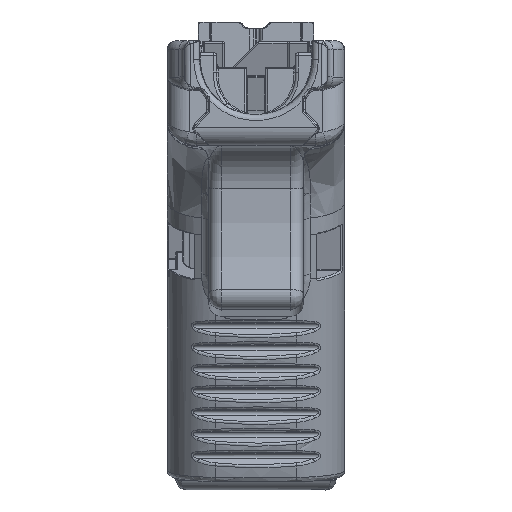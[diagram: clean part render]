
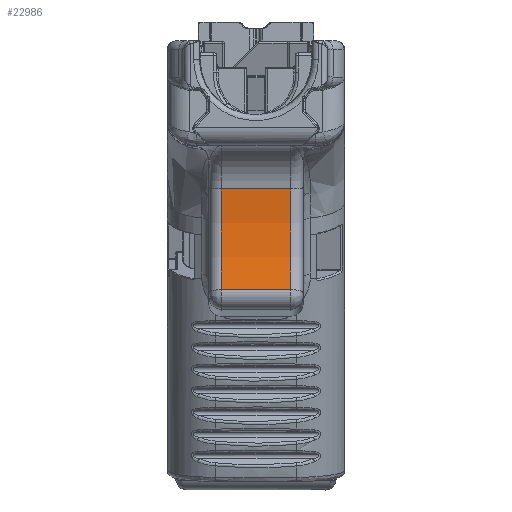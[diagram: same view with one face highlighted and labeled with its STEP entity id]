
A CAD part, top view. The second image highlights one B-rep face of the part: STEP entity #22986.
In plain terms, the highlighted cylindrical face has radius 41.155 mm (diameter 82.31 mm), a partial arc.
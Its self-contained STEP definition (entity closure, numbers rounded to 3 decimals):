
#2901=FACE_OUTER_BOUND('',#4463,.T.);
#4463=EDGE_LOOP('',(#17435,#17436,#17437,#17438));
#5932=LINE('',#53743,#7027);
#5933=LINE('',#53746,#7028);
#7027=VECTOR('',#29399,2.54);
#7028=VECTOR('',#29402,10.);
#8172=CIRCLE('',#25083,41.155);
#8173=CIRCLE('',#25084,41.155);
#9897=VERTEX_POINT('',#53739);
#9898=VERTEX_POINT('',#53740);
#9899=VERTEX_POINT('',#53742);
#9900=VERTEX_POINT('',#53744);
#12554=EDGE_CURVE('',#9897,#9898,#8172,.T.);
#12555=EDGE_CURVE('',#9899,#9897,#5932,.T.);
#12556=EDGE_CURVE('',#9900,#9899,#8173,.T.);
#12557=EDGE_CURVE('',#9898,#9900,#5933,.T.);
#17435=ORIENTED_EDGE('',*,*,#12554,.F.);
#17436=ORIENTED_EDGE('',*,*,#12555,.F.);
#17437=ORIENTED_EDGE('',*,*,#12556,.F.);
#17438=ORIENTED_EDGE('',*,*,#12557,.F.);
#22093=CYLINDRICAL_SURFACE('',#25082,41.155);
#22986=ADVANCED_FACE('',(#2901),#22093,.F.);
#25082=AXIS2_PLACEMENT_3D('',#53738,#29395,#29396);
#25083=AXIS2_PLACEMENT_3D('',#53741,#29397,#29398);
#25084=AXIS2_PLACEMENT_3D('',#53745,#29400,#29401);
#29395=DIRECTION('center_axis',(-1.,0.,0.));
#29396=DIRECTION('ref_axis',(0.,-0.291,-0.957));
#29397=DIRECTION('center_axis',(1.,0.,0.));
#29398=DIRECTION('ref_axis',(0.,-0.091,-0.996));
#29399=DIRECTION('',(-1.,0.,0.));
#29400=DIRECTION('center_axis',(-1.,0.,0.));
#29401=DIRECTION('ref_axis',(0.,-0.091,-0.996));
#29402=DIRECTION('',(1.,0.,0.));
#53738=CARTESIAN_POINT('Origin',(7.747,-29.007,0.864));
#53739=CARTESIAN_POINT('',(-5.747,-40.969,-38.514));
#53740=CARTESIAN_POINT('',(-5.747,-24.395,-40.032));
#53741=CARTESIAN_POINT('Origin',(-5.747,-29.007,0.864));
#53742=CARTESIAN_POINT('',(5.747,-40.969,-38.514));
#53743=CARTESIAN_POINT('',(7.747,-40.969,-38.514));
#53744=CARTESIAN_POINT('',(5.747,-24.395,-40.032));
#53745=CARTESIAN_POINT('Origin',(5.747,-29.007,0.864));
#53746=CARTESIAN_POINT('',(7.747,-24.395,-40.032));
